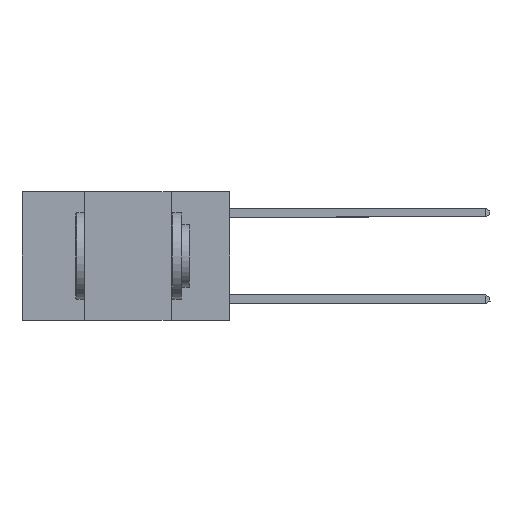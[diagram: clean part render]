
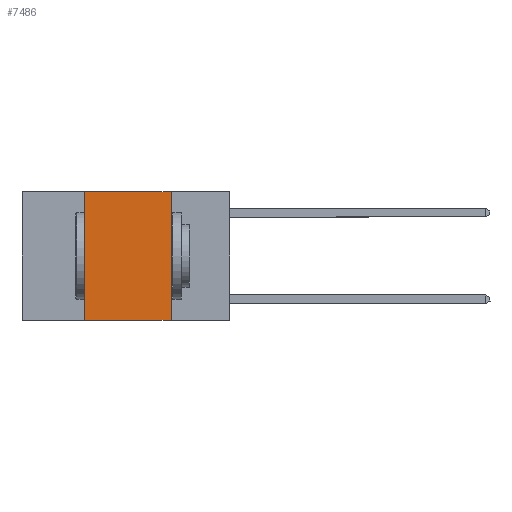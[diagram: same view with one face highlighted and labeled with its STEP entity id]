
A CAD part, left-side view. The second image highlights one B-rep face of the part: STEP entity #7486.
In plain terms, the highlighted planar face has unit normal (-1, 0, 0).
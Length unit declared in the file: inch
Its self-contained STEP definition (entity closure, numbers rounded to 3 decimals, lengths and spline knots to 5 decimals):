
#452 = CARTESIAN_POINT ( 'NONE',  ( 0., 0.17, 0. ) ) ;
#984 = ORIENTED_EDGE ( 'NONE', *, *, #9497, .T. ) ;
#1009 = CARTESIAN_POINT ( 'NONE',  ( 0., 0.6, 0. ) ) ;
#1253 = LINE ( 'NONE', #1358, #3486 ) ;
#1358 = CARTESIAN_POINT ( 'NONE',  ( 0., 0.6, 0. ) ) ;
#1649 = ORIENTED_EDGE ( 'NONE', *, *, #9480, .F. ) ;
#1854 = VERTEX_POINT ( 'NONE', #5148 ) ;
#1953 = EDGE_LOOP ( 'NONE', ( #7177, #1649, #10259, #984 ) ) ;
#1956 = DIRECTION ( 'NONE',  ( 0., 0., -1. ) ) ;
#2061 = CARTESIAN_POINT ( 'NONE',  ( 0., 0.17, 0. ) ) ;
#2331 = DIRECTION ( 'NONE',  ( 0., -1., 0. ) ) ;
#2851 = DIRECTION ( 'NONE',  ( 0., 0., 1. ) ) ;
#3486 = VECTOR ( 'NONE', #2331, 39.37008 ) ;
#3791 = AXIS2_PLACEMENT_3D ( 'NONE', #1009, #7498, #1956 ) ;
#3837 = VECTOR ( 'NONE', #5153, 39.37008 ) ;
#4230 = CARTESIAN_POINT ( 'NONE',  ( 0., 0.6, -0.37 ) ) ;
#5148 = CARTESIAN_POINT ( 'NONE',  ( 0., 0.42, 0. ) ) ;
#5153 = DIRECTION ( 'NONE',  ( 0., 0., -1. ) ) ;
#5174 = DIRECTION ( 'NONE',  ( 0., -1., 0. ) ) ;
#5676 = VECTOR ( 'NONE', #5174, 39.37008 ) ;
#5951 = LINE ( 'NONE', #4230, #5676 ) ;
#6084 = CARTESIAN_POINT ( 'NONE',  ( 0., 0.17, -0.37 ) ) ;
#6275 = CARTESIAN_POINT ( 'NONE',  ( 0., 0.42, -0.37 ) ) ;
#7036 = VERTEX_POINT ( 'NONE', #6084 ) ;
#7177 = ORIENTED_EDGE ( 'NONE', *, *, #10479, .F. ) ;
#7426 = EDGE_CURVE ( 'NONE', #10683, #1854, #9858, .T. ) ;
#7429 = CARTESIAN_POINT ( 'NONE',  ( 0., 0.42, 0. ) ) ;
#7486 = ADVANCED_FACE ( 'NONE', ( #8414 ), #10239, .F. ) ;
#7498 = DIRECTION ( 'NONE',  ( 1., 0., 0. ) ) ;
#8414 = FACE_OUTER_BOUND ( 'NONE', #1953, .T. ) ;
#8998 = VECTOR ( 'NONE', #2851, 39.37008 ) ;
#9480 = EDGE_CURVE ( 'NONE', #1854, #10282, #1253, .T. ) ;
#9497 = EDGE_CURVE ( 'NONE', #10683, #7036, #5951, .T. ) ;
#9858 = LINE ( 'NONE', #7429, #8998 ) ;
#10239 = PLANE ( 'NONE',  #3791 ) ;
#10259 = ORIENTED_EDGE ( 'NONE', *, *, #7426, .F. ) ;
#10282 = VERTEX_POINT ( 'NONE', #2061 ) ;
#10479 = EDGE_CURVE ( 'NONE', #10282, #7036, #11103, .T. ) ;
#10683 = VERTEX_POINT ( 'NONE', #6275 ) ;
#11103 = LINE ( 'NONE', #452, #3837 ) ;
